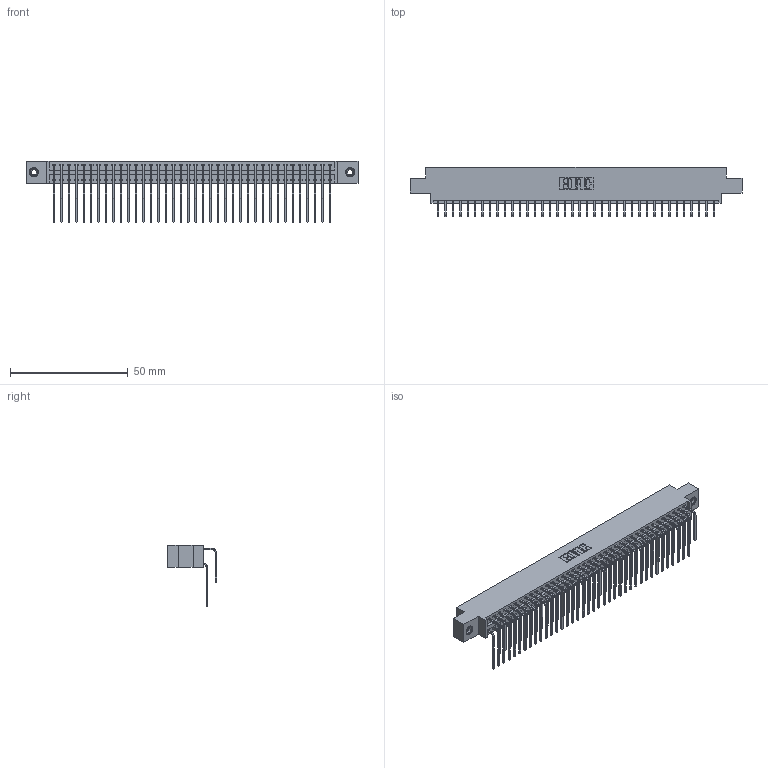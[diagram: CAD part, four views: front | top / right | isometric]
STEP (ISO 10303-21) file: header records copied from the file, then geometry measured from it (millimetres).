
FILE_DESCRIPTION (( 'STEP AP203' ), '1' );
FILE_NAME ('396-076-559-808.STEP', '2018-09-09T14:44:32', ( '' ), ( '' ), 'SwSTEP 2.0', 'SolidWorks 2016', '' );
FILE_SCHEMA (( 'CONFIG_CONTROL_DESIGN' ));
Length unit declared in the file: inch
Products named in the file (5): 345-250-001_345-250-003-102; 396-076-559-808; 346 Part_0.170 Offset - 0.156 Dia-TI; 345-292-001_558 559 Tail - 1; 345-292-001_559 Tail - 2
Assembly tree (79 placements, depth 2):
  396-076-559-808
    346 Part_0.170 Offset - 0.156 Dia-TI
    345-292-001_558 559 Tail - 1  x38
    345-292-001_559 Tail - 2  x38
    345-250-001_345-250-003-102  x2
Bounding box: 141.22 x 20.89 x 26.16 mm (x, y, z)
Volume: 14017.3 mm3; surface area: 21507.8 mm2
Topology: 79 solids, 79 shells, 4290 faces, 12713 edges, 8366 vertices
Faces by surface type: plane 2924, cylinder 1350, cone 12, torus 4
Entity records: 28440 total; most frequent: CARTESIAN_POINT 4730, ORIENTED_EDGE 4606, DIRECTION 4217, EDGE_CURVE 2303, VECTOR 1959, LINE 1959, VERTEX_POINT 1528, AXIS2_PLACEMENT_3D 1129
